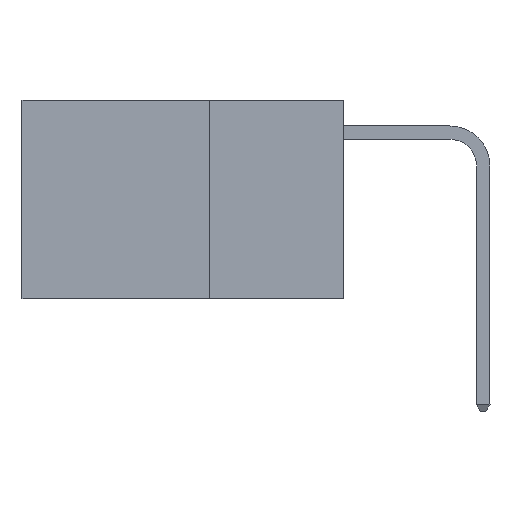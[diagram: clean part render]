
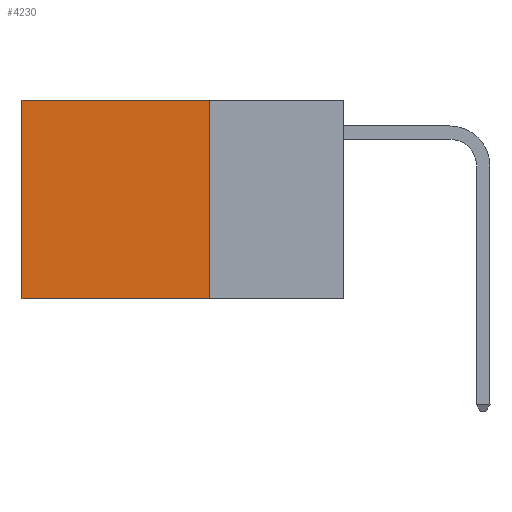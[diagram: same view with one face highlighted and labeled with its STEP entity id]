
A CAD part, left-side view. The second image highlights one B-rep face of the part: STEP entity #4230.
In plain terms, the highlighted planar face has unit normal (-1, 0, 0).
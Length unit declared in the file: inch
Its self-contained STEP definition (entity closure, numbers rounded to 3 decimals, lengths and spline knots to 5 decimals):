
#13 = CARTESIAN_POINT ( 'NONE',  ( 0.2625, 0.25, -0.37 ) ) ;
#518 = EDGE_CURVE ( 'NONE', #1680, #766, #2972, .T. ) ;
#766 = VERTEX_POINT ( 'NONE', #6026 ) ;
#1264 = VECTOR ( 'NONE', #2036, 39.37008 ) ;
#1284 = LINE ( 'NONE', #2049, #1264 ) ;
#1680 = VERTEX_POINT ( 'NONE', #5590 ) ;
#1847 = DIRECTION ( 'NONE',  ( 0., 0., -1. ) ) ;
#1893 = CARTESIAN_POINT ( 'NONE',  ( 0.2625, 0.6, 0. ) ) ;
#2036 = DIRECTION ( 'NONE',  ( 0., 1., 0. ) ) ;
#2049 = CARTESIAN_POINT ( 'NONE',  ( 0.2625, 0.25, 0. ) ) ;
#2551 = EDGE_CURVE ( 'NONE', #7377, #766, #11282, .T. ) ;
#2711 = DIRECTION ( 'NONE',  ( 1., 0., 0. ) ) ;
#2806 = DIRECTION ( 'NONE',  ( 0., 1., 0. ) ) ;
#2940 = VECTOR ( 'NONE', #2806, 39.37008 ) ;
#2972 = LINE ( 'NONE', #13, #2940 ) ;
#3381 = PLANE ( 'NONE',  #5214 ) ;
#3669 = CARTESIAN_POINT ( 'NONE',  ( 0.2625, 0.25, 0. ) ) ;
#3674 = VECTOR ( 'NONE', #11546, 39.37008 ) ;
#3746 = LINE ( 'NONE', #11309, #3674 ) ;
#4230 = ADVANCED_FACE ( 'NONE', ( #4376 ), #3381, .F. ) ;
#4301 = EDGE_LOOP ( 'NONE', ( #6074, #6406, #6799, #7284 ) ) ;
#4376 = FACE_OUTER_BOUND ( 'NONE', #4301, .T. ) ;
#5214 = AXIS2_PLACEMENT_3D ( 'NONE', #10542, #2711, #7642 ) ;
#5590 = CARTESIAN_POINT ( 'NONE',  ( 0.2625, 0.25, -0.37 ) ) ;
#6026 = CARTESIAN_POINT ( 'NONE',  ( 0.2625, 0.6, -0.37 ) ) ;
#6074 = ORIENTED_EDGE ( 'NONE', *, *, #2551, .T. ) ;
#6406 = ORIENTED_EDGE ( 'NONE', *, *, #518, .F. ) ;
#6799 = ORIENTED_EDGE ( 'NONE', *, *, #9242, .F. ) ;
#7284 = ORIENTED_EDGE ( 'NONE', *, *, #10591, .T. ) ;
#7377 = VERTEX_POINT ( 'NONE', #9875 ) ;
#7642 = DIRECTION ( 'NONE',  ( 0., 0., -1. ) ) ;
#8110 = VERTEX_POINT ( 'NONE', #3669 ) ;
#9242 = EDGE_CURVE ( 'NONE', #8110, #1680, #3746, .T. ) ;
#9875 = CARTESIAN_POINT ( 'NONE',  ( 0.2625, 0.6, 0. ) ) ;
#10542 = CARTESIAN_POINT ( 'NONE',  ( 0.2625, 0.25, 0. ) ) ;
#10591 = EDGE_CURVE ( 'NONE', #8110, #7377, #1284, .T. ) ;
#11260 = VECTOR ( 'NONE', #1847, 39.37008 ) ;
#11282 = LINE ( 'NONE', #1893, #11260 ) ;
#11309 = CARTESIAN_POINT ( 'NONE',  ( 0.2625, 0.25, 0. ) ) ;
#11546 = DIRECTION ( 'NONE',  ( 0., 0., -1. ) ) ;
